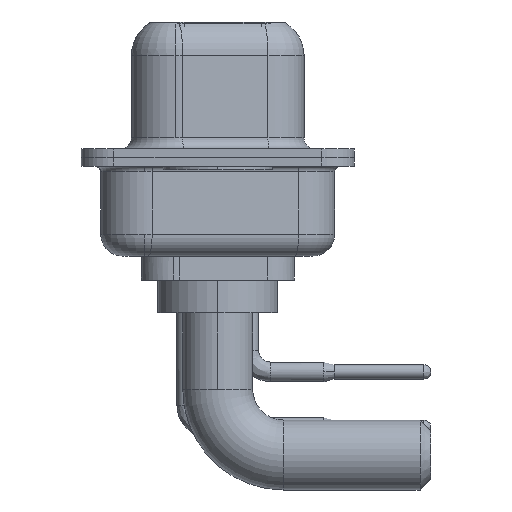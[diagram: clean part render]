
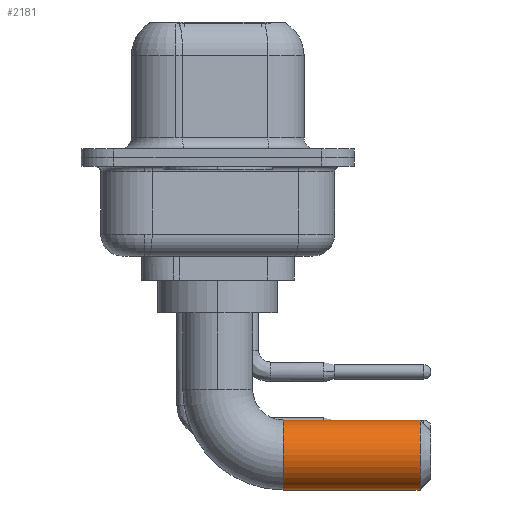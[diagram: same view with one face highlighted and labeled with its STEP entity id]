
A CAD part, left-side view. The second image highlights one B-rep face of the part: STEP entity #2181.
In plain terms, the highlighted cylindrical face has radius 1.6 mm (diameter 3.2 mm), a partial arc.
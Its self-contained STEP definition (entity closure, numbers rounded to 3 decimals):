
#71 = VERTEX_POINT ( 'NONE', #3690 ) ;
#245 = ORIENTED_EDGE ( 'NONE', *, *, #4987, .F. ) ;
#1053 = EDGE_CURVE ( 'NONE', #3208, #2942, #5755, .T. ) ;
#1105 = CARTESIAN_POINT ( 'NONE',  ( 0., -9.25, -6.5 ) ) ;
#1675 = DIRECTION ( 'NONE',  ( 0., -1., 0. ) ) ;
#1999 = CARTESIAN_POINT ( 'NONE',  ( 0., -3., -4.9 ) ) ;
#2181 = ADVANCED_FACE ( 'NONE', ( #12500 ), #8913, .T. ) ;
#2942 = VERTEX_POINT ( 'NONE', #13688 ) ;
#3112 = DIRECTION ( 'NONE',  ( 0., -1., 0. ) ) ;
#3208 = VERTEX_POINT ( 'NONE', #12284 ) ;
#3388 = ORIENTED_EDGE ( 'NONE', *, *, #1053, .T. ) ;
#3690 = CARTESIAN_POINT ( 'NONE',  ( 0., -3., -8.1 ) ) ;
#3773 = CARTESIAN_POINT ( 'NONE',  ( 0., -3., -4.9 ) ) ;
#4470 = VERTEX_POINT ( 'NONE', #3773 ) ;
#4987 = EDGE_CURVE ( 'NONE', #4470, #2942, #9383, .T. ) ;
#5755 = CIRCLE ( 'NONE', #9253, 1.6 ) ;
#5964 = VECTOR ( 'NONE', #12155, 1000. ) ;
#6936 = AXIS2_PLACEMENT_3D ( 'NONE', #6943, #10620, #11712 ) ;
#6943 = CARTESIAN_POINT ( 'NONE',  ( 0., -3., -6.5 ) ) ;
#7319 = DIRECTION ( 'NONE',  ( 0., 1., 0. ) ) ;
#7494 = AXIS2_PLACEMENT_3D ( 'NONE', #12735, #1675, #9067 ) ;
#7741 = ORIENTED_EDGE ( 'NONE', *, *, #14477, .T. ) ;
#8913 = CYLINDRICAL_SURFACE ( 'NONE', #7494, 1.6 ) ;
#8931 = LINE ( 'NONE', #13246, #5964 ) ;
#9067 = DIRECTION ( 'NONE',  ( 0., 0., -1. ) ) ;
#9253 = AXIS2_PLACEMENT_3D ( 'NONE', #1105, #7319, #11928 ) ;
#9383 = LINE ( 'NONE', #1999, #13549 ) ;
#10620 = DIRECTION ( 'NONE',  ( 0., -1., 0. ) ) ;
#11712 = DIRECTION ( 'NONE',  ( -1., 0., 0. ) ) ;
#11928 = DIRECTION ( 'NONE',  ( 0., 0., -1. ) ) ;
#12149 = EDGE_CURVE ( 'NONE', #4470, #71, #12671, .T. ) ;
#12155 = DIRECTION ( 'NONE',  ( 0., -1., 0. ) ) ;
#12284 = CARTESIAN_POINT ( 'NONE',  ( 0., -9.25, -8.1 ) ) ;
#12500 = FACE_OUTER_BOUND ( 'NONE', #12798, .T. ) ;
#12671 = CIRCLE ( 'NONE', #6936, 1.6 ) ;
#12735 = CARTESIAN_POINT ( 'NONE',  ( 0., -3., -6.5 ) ) ;
#12798 = EDGE_LOOP ( 'NONE', ( #245, #13805, #7741, #3388 ) ) ;
#13246 = CARTESIAN_POINT ( 'NONE',  ( 0., -3., -8.1 ) ) ;
#13549 = VECTOR ( 'NONE', #3112, 1000. ) ;
#13688 = CARTESIAN_POINT ( 'NONE',  ( 0., -9.25, -4.9 ) ) ;
#13805 = ORIENTED_EDGE ( 'NONE', *, *, #12149, .T. ) ;
#14477 = EDGE_CURVE ( 'NONE', #71, #3208, #8931, .T. ) ;
